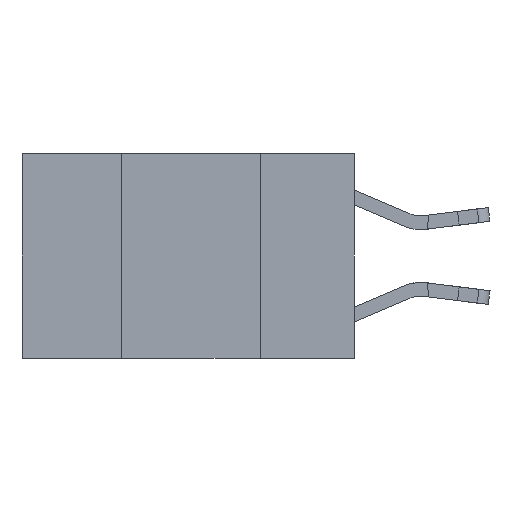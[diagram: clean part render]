
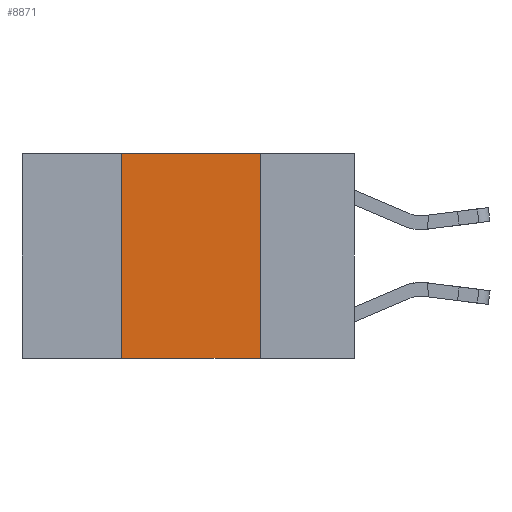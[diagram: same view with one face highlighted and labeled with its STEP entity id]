
A CAD part, left-side view. The second image highlights one B-rep face of the part: STEP entity #8871.
In plain terms, the highlighted planar face has unit normal (-1, 0, 0).
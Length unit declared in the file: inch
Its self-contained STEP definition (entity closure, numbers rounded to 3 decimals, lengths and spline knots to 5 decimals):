
#228 = CARTESIAN_POINT ( 'NONE',  ( 0., 0.6, -0.37 ) ) ;
#979 = VECTOR ( 'NONE', #2457, 39.37008 ) ;
#2173 = ORIENTED_EDGE ( 'NONE', *, *, #20033, .T. ) ;
#2457 = DIRECTION ( 'NONE',  ( 0., 0., -1. ) ) ;
#2726 = FACE_OUTER_BOUND ( 'NONE', #14953, .T. ) ;
#4547 = DIRECTION ( 'NONE',  ( 0., 0., 1. ) ) ;
#5635 = LINE ( 'NONE', #19720, #16546 ) ;
#6323 = VERTEX_POINT ( 'NONE', #12396 ) ;
#6359 = VERTEX_POINT ( 'NONE', #21116 ) ;
#6850 = CARTESIAN_POINT ( 'NONE',  ( 0., 0.42, -0.37 ) ) ;
#8871 = ADVANCED_FACE ( 'NONE', ( #2726 ), #9535, .F. ) ;
#9116 = VERTEX_POINT ( 'NONE', #21357 ) ;
#9535 = PLANE ( 'NONE',  #24643 ) ;
#9939 = EDGE_CURVE ( 'NONE', #15436, #6359, #10196, .T. ) ;
#10196 = LINE ( 'NONE', #26000, #20291 ) ;
#11394 = EDGE_CURVE ( 'NONE', #9116, #6323, #18329, .T. ) ;
#11700 = DIRECTION ( 'NONE',  ( 0., 0., -1. ) ) ;
#11739 = ORIENTED_EDGE ( 'NONE', *, *, #11394, .F. ) ;
#12396 = CARTESIAN_POINT ( 'NONE',  ( 0., 0.17, -0.37 ) ) ;
#12423 = ORIENTED_EDGE ( 'NONE', *, *, #9939, .F. ) ;
#14953 = EDGE_LOOP ( 'NONE', ( #11739, #23142, #12423, #2173 ) ) ;
#15436 = VERTEX_POINT ( 'NONE', #6850 ) ;
#15492 = DIRECTION ( 'NONE',  ( 0., -1., 0. ) ) ;
#16546 = VECTOR ( 'NONE', #21866, 39.37008 ) ;
#16865 = LINE ( 'NONE', #228, #17536 ) ;
#17536 = VECTOR ( 'NONE', #15492, 39.37008 ) ;
#18329 = LINE ( 'NONE', #19721, #979 ) ;
#19332 = EDGE_CURVE ( 'NONE', #6359, #9116, #5635, .T. ) ;
#19720 = CARTESIAN_POINT ( 'NONE',  ( 0., 0.6, 0. ) ) ;
#19721 = CARTESIAN_POINT ( 'NONE',  ( 0., 0.17, 0. ) ) ;
#20033 = EDGE_CURVE ( 'NONE', #15436, #6323, #16865, .T. ) ;
#20291 = VECTOR ( 'NONE', #4547, 39.37008 ) ;
#21116 = CARTESIAN_POINT ( 'NONE',  ( 0., 0.42, 0. ) ) ;
#21357 = CARTESIAN_POINT ( 'NONE',  ( 0., 0.17, 0. ) ) ;
#21866 = DIRECTION ( 'NONE',  ( 0., -1., 0. ) ) ;
#22389 = CARTESIAN_POINT ( 'NONE',  ( 0., 0.6, 0. ) ) ;
#23142 = ORIENTED_EDGE ( 'NONE', *, *, #19332, .F. ) ;
#24536 = DIRECTION ( 'NONE',  ( 1., 0., 0. ) ) ;
#24643 = AXIS2_PLACEMENT_3D ( 'NONE', #22389, #24536, #11700 ) ;
#26000 = CARTESIAN_POINT ( 'NONE',  ( 0., 0.42, 0. ) ) ;
